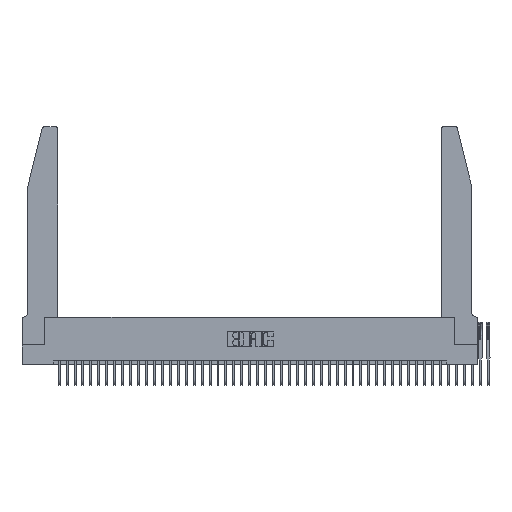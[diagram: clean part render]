
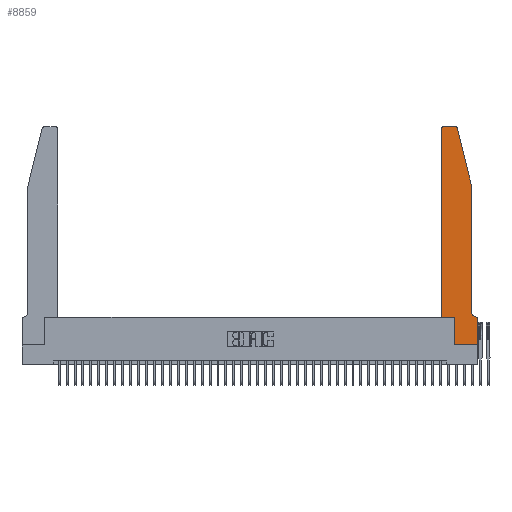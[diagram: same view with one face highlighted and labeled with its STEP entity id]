
A CAD part, top view. The second image highlights one B-rep face of the part: STEP entity #8859.
In plain terms, the highlighted face is planar.
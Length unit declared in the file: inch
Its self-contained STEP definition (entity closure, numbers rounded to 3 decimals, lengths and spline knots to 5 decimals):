
#16 = VERTEX_POINT ( 'NONE', #2922 ) ;
#48 = CARTESIAN_POINT ( 'NONE',  ( 0.2865, 0.35, 0. ) ) ;
#455 = EDGE_CURVE ( 'NONE', #31619, #6109, #34085, .T. ) ;
#528 = EDGE_CURVE ( 'NONE', #4903, #22419, #4869, .T. ) ;
#618 = AXIS2_PLACEMENT_3D ( 'NONE', #18405, #40153, #21605 ) ;
#977 = EDGE_CURVE ( 'NONE', #29257, #27345, #24278, .T. ) ;
#1581 = CARTESIAN_POINT ( 'NONE',  ( 0.0755, 0.42, 0. ) ) ;
#1906 = ORIENTED_EDGE ( 'NONE', *, *, #528, .F. ) ;
#2167 = CARTESIAN_POINT ( 'NONE',  ( 0.4505, 0.35, 0. ) ) ;
#2381 = ORIENTED_EDGE ( 'NONE', *, *, #19879, .T. ) ;
#2427 = CARTESIAN_POINT ( 'NONE',  ( 0.0755, 2., 0. ) ) ;
#2464 = LINE ( 'NONE', #5189, #37079 ) ;
#2922 = CARTESIAN_POINT ( 'NONE',  ( 0., 0., 0. ) ) ;
#3896 = CARTESIAN_POINT ( 'NONE',  ( 0., 0.35, 0. ) ) ;
#4034 = PLANE ( 'NONE',  #34005 ) ;
#4059 = ORIENTED_EDGE ( 'NONE', *, *, #8416, .F. ) ;
#4226 = VERTEX_POINT ( 'NONE', #1581 ) ;
#4291 = ORIENTED_EDGE ( 'NONE', *, *, #455, .F. ) ;
#4813 = VERTEX_POINT ( 'NONE', #39110 ) ;
#4869 = LINE ( 'NONE', #40636, #14445 ) ;
#4903 = VERTEX_POINT ( 'NONE', #29029 ) ;
#5189 = CARTESIAN_POINT ( 'NONE',  ( 0., 0., 0. ) ) ;
#5496 = CARTESIAN_POINT ( 'NONE',  ( 0.0755, 0.35, 0. ) ) ;
#6109 = VERTEX_POINT ( 'NONE', #18974 ) ;
#6170 = EDGE_LOOP ( 'NONE', ( #1906, #9772, #40470, #2381, #26009, #4291, #10090, #21857, #4059, #7327, #24645, #26087 ) ) ;
#7260 = DIRECTION ( 'NONE',  ( 0., 0., 1. ) ) ;
#7327 = ORIENTED_EDGE ( 'NONE', *, *, #977, .F. ) ;
#7582 = CARTESIAN_POINT ( 'NONE',  ( 0.2865, 0.35, 0. ) ) ;
#8416 = EDGE_CURVE ( 'NONE', #27345, #16, #2464, .T. ) ;
#8433 = DIRECTION ( 'NONE',  ( 0., -1., 0. ) ) ;
#8675 = VECTOR ( 'NONE', #19181, 39.37008 ) ;
#8859 = ADVANCED_FACE ( 'NONE', ( #20526 ), #4034, .F. ) ;
#8886 = VECTOR ( 'NONE', #27045, 39.37008 ) ;
#8940 = LINE ( 'NONE', #26613, #32180 ) ;
#9246 = CARTESIAN_POINT ( 'NONE',  ( 0.4205, 2.75, 0. ) ) ;
#9348 = EDGE_CURVE ( 'NONE', #16, #4813, #8940, .T. ) ;
#9772 = ORIENTED_EDGE ( 'NONE', *, *, #17738, .T. ) ;
#10090 = ORIENTED_EDGE ( 'NONE', *, *, #13663, .F. ) ;
#10799 = DIRECTION ( 'NONE',  ( 1., 0., 0. ) ) ;
#11742 = DIRECTION ( 'NONE',  ( 1., 0., 0. ) ) ;
#11968 = VERTEX_POINT ( 'NONE', #14216 ) ;
#12695 = CARTESIAN_POINT ( 'NONE',  ( 0., 0.35, 0. ) ) ;
#13062 = CARTESIAN_POINT ( 'NONE',  ( 0.0755, 2., 0. ) ) ;
#13204 = CARTESIAN_POINT ( 'NONE',  ( 0.284, 2.72, 0. ) ) ;
#13254 = VECTOR ( 'NONE', #31956, 39.37008 ) ;
#13314 = VERTEX_POINT ( 'NONE', #17177 ) ;
#13663 = EDGE_CURVE ( 'NONE', #4813, #31619, #32978, .T. ) ;
#14216 = CARTESIAN_POINT ( 'NONE',  ( 0.284, 2.75, 0. ) ) ;
#14445 = VECTOR ( 'NONE', #28078, 39.37008 ) ;
#14934 = AXIS2_PLACEMENT_3D ( 'NONE', #13204, #35176, #16473 ) ;
#16165 = DIRECTION ( 'NONE',  ( 0., 1., 0. ) ) ;
#16259 = CIRCLE ( 'NONE', #618, 0.03 ) ;
#16317 = VECTOR ( 'NONE', #16165, 39.37008 ) ;
#16473 = DIRECTION ( 'NONE',  ( 1., 0., 0. ) ) ;
#17177 = CARTESIAN_POINT ( 'NONE',  ( 0.4505, 2.72, 0. ) ) ;
#17544 = DIRECTION ( 'NONE',  ( 0., 0., -1. ) ) ;
#17738 = EDGE_CURVE ( 'NONE', #4903, #11968, #34604, .T. ) ;
#18405 = CARTESIAN_POINT ( 'NONE',  ( 0.4205, 2.72, 0. ) ) ;
#18450 = DIRECTION ( 'NONE',  ( -1., 0., 0. ) ) ;
#18481 = VECTOR ( 'NONE', #11742, 39.37008 ) ;
#18974 = CARTESIAN_POINT ( 'NONE',  ( 0.4505, 0.35, 0. ) ) ;
#19025 = CARTESIAN_POINT ( 'NONE',  ( 0.0055, 0.35, 0. ) ) ;
#19181 = DIRECTION ( 'NONE',  ( 0., 1., 0. ) ) ;
#19486 = EDGE_CURVE ( 'NONE', #22419, #4226, #30050, .T. ) ;
#19879 = EDGE_CURVE ( 'NONE', #30457, #13314, #16259, .T. ) ;
#20313 = EDGE_CURVE ( 'NONE', #6109, #13314, #33848, .T. ) ;
#20526 = FACE_OUTER_BOUND ( 'NONE', #6170, .T. ) ;
#21605 = DIRECTION ( 'NONE',  ( 1., 0., 0. ) ) ;
#21857 = ORIENTED_EDGE ( 'NONE', *, *, #9348, .F. ) ;
#22419 = VERTEX_POINT ( 'NONE', #2427 ) ;
#23571 = EDGE_CURVE ( 'NONE', #4226, #29257, #39855, .T. ) ;
#23925 = CARTESIAN_POINT ( 'NONE',  ( 0.2605, 2.75, 0. ) ) ;
#24278 = LINE ( 'NONE', #5496, #31548 ) ;
#24645 = ORIENTED_EDGE ( 'NONE', *, *, #23571, .F. ) ;
#24994 = CARTESIAN_POINT ( 'NONE',  ( 0.4505, 0.35, 0. ) ) ;
#25839 = LINE ( 'NONE', #23925, #8886 ) ;
#26009 = ORIENTED_EDGE ( 'NONE', *, *, #20313, .F. ) ;
#26087 = ORIENTED_EDGE ( 'NONE', *, *, #19486, .F. ) ;
#26613 = CARTESIAN_POINT ( 'NONE',  ( 0., 0., 0. ) ) ;
#27045 = DIRECTION ( 'NONE',  ( -1., 0., 0. ) ) ;
#27345 = VERTEX_POINT ( 'NONE', #12695 ) ;
#28078 = DIRECTION ( 'NONE',  ( -0.239, -0.971, 0. ) ) ;
#29029 = CARTESIAN_POINT ( 'NONE',  ( 0.25487, 2.72718, 0. ) ) ;
#29257 = VERTEX_POINT ( 'NONE', #19025 ) ;
#29465 = DIRECTION ( 'NONE',  ( 1., 0., 0. ) ) ;
#30050 = LINE ( 'NONE', #13062, #13254 ) ;
#30181 = EDGE_CURVE ( 'NONE', #30457, #11968, #25839, .T. ) ;
#30457 = VERTEX_POINT ( 'NONE', #9246 ) ;
#31126 = AXIS2_PLACEMENT_3D ( 'NONE', #36204, #17544, #39323 ) ;
#31548 = VECTOR ( 'NONE', #18450, 39.37008 ) ;
#31619 = VERTEX_POINT ( 'NONE', #7582 ) ;
#31956 = DIRECTION ( 'NONE',  ( 0., -1., 0. ) ) ;
#32180 = VECTOR ( 'NONE', #10799, 39.37008 ) ;
#32978 = LINE ( 'NONE', #48, #16317 ) ;
#33848 = LINE ( 'NONE', #24994, #8675 ) ;
#34005 = AXIS2_PLACEMENT_3D ( 'NONE', #3896, #7260, #29465 ) ;
#34085 = LINE ( 'NONE', #2167, #18481 ) ;
#34604 = CIRCLE ( 'NONE', #14934, 0.03 ) ;
#35176 = DIRECTION ( 'NONE',  ( 0., 0., -1. ) ) ;
#36204 = CARTESIAN_POINT ( 'NONE',  ( 0.0055, 0.42, 0. ) ) ;
#37079 = VECTOR ( 'NONE', #8433, 39.37008 ) ;
#39110 = CARTESIAN_POINT ( 'NONE',  ( 0.2865, 0., 0. ) ) ;
#39323 = DIRECTION ( 'NONE',  ( -1., 0., 0. ) ) ;
#39855 = CIRCLE ( 'NONE', #31126, 0.07 ) ;
#40153 = DIRECTION ( 'NONE',  ( 0., 0., -1. ) ) ;
#40470 = ORIENTED_EDGE ( 'NONE', *, *, #30181, .F. ) ;
#40636 = CARTESIAN_POINT ( 'NONE',  ( 0.0755, 2., 0. ) ) ;
